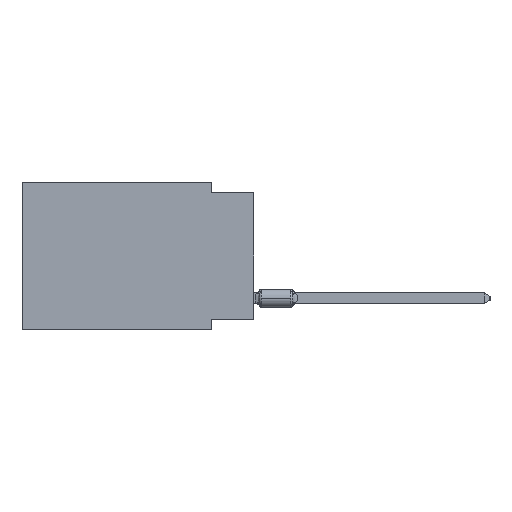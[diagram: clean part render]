
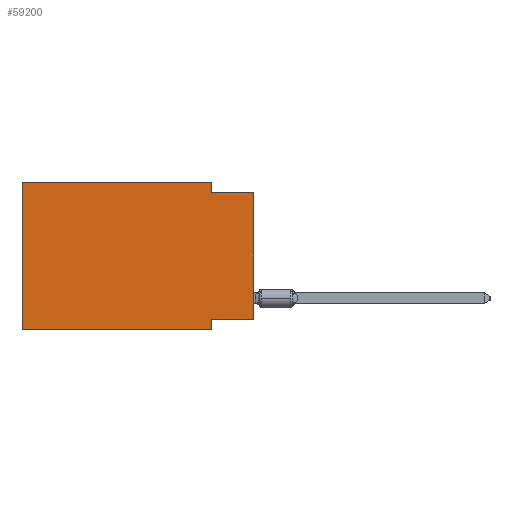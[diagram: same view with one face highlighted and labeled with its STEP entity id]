
A CAD part, left-side view. The second image highlights one B-rep face of the part: STEP entity #59200.
In plain terms, the highlighted planar face has unit normal (-1, 0, 0).
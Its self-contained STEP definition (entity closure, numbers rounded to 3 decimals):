
#1188 = VECTOR ( 'NONE', #40908, 1000. ) ;
#1815 = DIRECTION ( 'NONE',  ( 0., -1., 0. ) ) ;
#2007 = FACE_OUTER_BOUND ( 'NONE', #29353, .T. ) ;
#3117 = ORIENTED_EDGE ( 'NONE', *, *, #12892, .F. ) ;
#4050 = VERTEX_POINT ( 'NONE', #34351 ) ;
#4201 = VECTOR ( 'NONE', #21923, 1000. ) ;
#6933 = LINE ( 'NONE', #17141, #4201 ) ;
#7409 = CARTESIAN_POINT ( 'NONE',  ( 0., 0., -8.255 ) ) ;
#9062 = EDGE_CURVE ( 'NONE', #26984, #14823, #28420, .T. ) ;
#10206 = DIRECTION ( 'NONE',  ( 0., 0., -1. ) ) ;
#12892 = EDGE_CURVE ( 'NONE', #18216, #32211, #55411, .T. ) ;
#13884 = VECTOR ( 'NONE', #60542, 1000. ) ;
#14235 = EDGE_CURVE ( 'NONE', #19197, #32211, #21405, .T. ) ;
#14823 = VERTEX_POINT ( 'NONE', #61621 ) ;
#16925 = VECTOR ( 'NONE', #22086, 1000. ) ;
#17141 = CARTESIAN_POINT ( 'NONE',  ( 0., 0., -0.635 ) ) ;
#18216 = VERTEX_POINT ( 'NONE', #31367 ) ;
#19004 = EDGE_CURVE ( 'NONE', #57297, #26984, #40197, .T. ) ;
#19197 = VERTEX_POINT ( 'NONE', #42945 ) ;
#19454 = CARTESIAN_POINT ( 'NONE',  ( 0., 0., -8.255 ) ) ;
#20179 = EDGE_CURVE ( 'NONE', #43889, #18216, #32312, .T. ) ;
#21014 = CARTESIAN_POINT ( 'NONE',  ( 0., 13.97, 0. ) ) ;
#21405 = LINE ( 'NONE', #21713, #1188 ) ;
#21713 = CARTESIAN_POINT ( 'NONE',  ( 0., 13.97, -8.89 ) ) ;
#21812 = PLANE ( 'NONE',  #61279 ) ;
#21923 = DIRECTION ( 'NONE',  ( 0., -1., 0. ) ) ;
#21990 = LINE ( 'NONE', #36706, #60829 ) ;
#22086 = DIRECTION ( 'NONE',  ( 0., 1., 0. ) ) ;
#22271 = ORIENTED_EDGE ( 'NONE', *, *, #14235, .T. ) ;
#22547 = ORIENTED_EDGE ( 'NONE', *, *, #54484, .F. ) ;
#23065 = CARTESIAN_POINT ( 'NONE',  ( 0., 0., 0. ) ) ;
#24887 = CARTESIAN_POINT ( 'NONE',  ( 0., 2.54, 0. ) ) ;
#26984 = VERTEX_POINT ( 'NONE', #60579 ) ;
#28420 = LINE ( 'NONE', #24887, #34025 ) ;
#29034 = ORIENTED_EDGE ( 'NONE', *, *, #9062, .F. ) ;
#29353 = EDGE_LOOP ( 'NONE', ( #46840, #36921, #29034, #56127, #22547, #22271, #3117, #42205 ) ) ;
#31367 = CARTESIAN_POINT ( 'NONE',  ( 0., 2.54, -8.255 ) ) ;
#32211 = VERTEX_POINT ( 'NONE', #53060 ) ;
#32312 = LINE ( 'NONE', #7409, #16925 ) ;
#34025 = VECTOR ( 'NONE', #10206, 1000. ) ;
#34351 = CARTESIAN_POINT ( 'NONE',  ( 0., 0., -0.635 ) ) ;
#35306 = VECTOR ( 'NONE', #1815, 1000. ) ;
#36706 = CARTESIAN_POINT ( 'NONE',  ( 0., 13.97, 0. ) ) ;
#36921 = ORIENTED_EDGE ( 'NONE', *, *, #48210, .F. ) ;
#40197 = LINE ( 'NONE', #21014, #35306 ) ;
#40692 = CARTESIAN_POINT ( 'NONE',  ( 0., 13.97, 0. ) ) ;
#40908 = DIRECTION ( 'NONE',  ( 0., -1., 0. ) ) ;
#42205 = ORIENTED_EDGE ( 'NONE', *, *, #20179, .F. ) ;
#42945 = CARTESIAN_POINT ( 'NONE',  ( 0., 13.97, -8.89 ) ) ;
#43889 = VERTEX_POINT ( 'NONE', #19454 ) ;
#46840 = ORIENTED_EDGE ( 'NONE', *, *, #60576, .T. ) ;
#47060 = VECTOR ( 'NONE', #57329, 1000. ) ;
#48023 = LINE ( 'NONE', #23065, #47060 ) ;
#48210 = EDGE_CURVE ( 'NONE', #14823, #4050, #6933, .T. ) ;
#50596 = CARTESIAN_POINT ( 'NONE',  ( 0., 2.54, -8.89 ) ) ;
#53060 = CARTESIAN_POINT ( 'NONE',  ( 0., 2.54, -8.89 ) ) ;
#54484 = EDGE_CURVE ( 'NONE', #19197, #57297, #21990, .T. ) ;
#55112 = DIRECTION ( 'NONE',  ( 1., 0., 0. ) ) ;
#55411 = LINE ( 'NONE', #50596, #13884 ) ;
#55907 = DIRECTION ( 'NONE',  ( 0., 0., 1. ) ) ;
#56127 = ORIENTED_EDGE ( 'NONE', *, *, #19004, .F. ) ;
#57297 = VERTEX_POINT ( 'NONE', #40692 ) ;
#57329 = DIRECTION ( 'NONE',  ( 0., 0., 1. ) ) ;
#59200 = ADVANCED_FACE ( 'NONE', ( #2007 ), #21812, .F. ) ;
#59916 = DIRECTION ( 'NONE',  ( 0., 0., -1. ) ) ;
#60542 = DIRECTION ( 'NONE',  ( 0., 0., -1. ) ) ;
#60557 = CARTESIAN_POINT ( 'NONE',  ( 0., 13.97, 0. ) ) ;
#60576 = EDGE_CURVE ( 'NONE', #43889, #4050, #48023, .T. ) ;
#60579 = CARTESIAN_POINT ( 'NONE',  ( 0., 2.54, 0. ) ) ;
#60829 = VECTOR ( 'NONE', #55907, 1000. ) ;
#61279 = AXIS2_PLACEMENT_3D ( 'NONE', #60557, #55112, #59916 ) ;
#61621 = CARTESIAN_POINT ( 'NONE',  ( 0., 2.54, -0.635 ) ) ;
